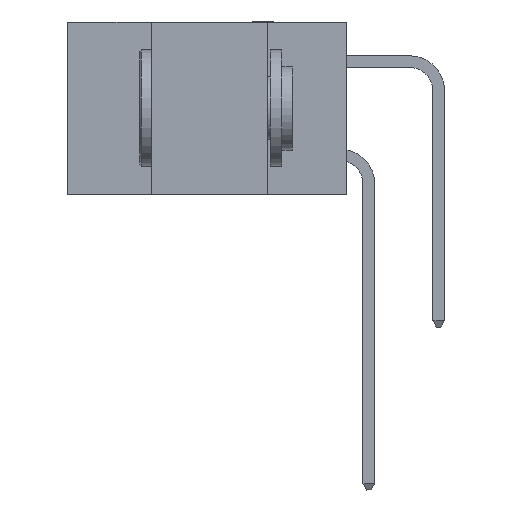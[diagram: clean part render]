
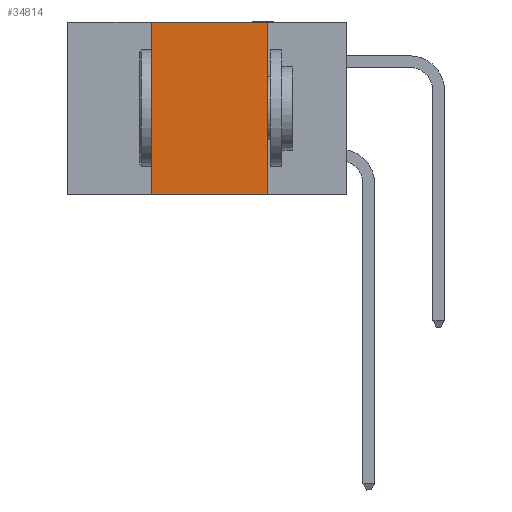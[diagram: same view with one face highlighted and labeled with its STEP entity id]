
A CAD part, left-side view. The second image highlights one B-rep face of the part: STEP entity #34814.
In plain terms, the highlighted planar face has unit normal (-1, 0, 0).
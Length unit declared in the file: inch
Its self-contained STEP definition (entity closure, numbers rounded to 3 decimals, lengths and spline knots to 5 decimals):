
#4759 = CARTESIAN_POINT ( 'NONE',  ( 0., 0.42, -0.37 ) ) ;
#5183 = VERTEX_POINT ( 'NONE', #14195 ) ;
#7444 = EDGE_CURVE ( 'NONE', #23126, #5183, #34120, .T. ) ;
#9278 = ORIENTED_EDGE ( 'NONE', *, *, #34131, .T. ) ;
#10661 = ORIENTED_EDGE ( 'NONE', *, *, #11235, .F. ) ;
#11235 = EDGE_CURVE ( 'NONE', #43028, #21261, #43667, .T. ) ;
#12449 = CARTESIAN_POINT ( 'NONE',  ( 0., 0.6, -0.37 ) ) ;
#12521 = CARTESIAN_POINT ( 'NONE',  ( 0., 0.6, 0. ) ) ;
#12543 = ORIENTED_EDGE ( 'NONE', *, *, #41556, .F. ) ;
#12591 = DIRECTION ( 'NONE',  ( 0., -1., 0. ) ) ;
#14195 = CARTESIAN_POINT ( 'NONE',  ( 0., 0.42, 0. ) ) ;
#14904 = LINE ( 'NONE', #12449, #32244 ) ;
#15912 = PLANE ( 'NONE',  #23015 ) ;
#16789 = VECTOR ( 'NONE', #43721, 39.37008 ) ;
#19611 = CARTESIAN_POINT ( 'NONE',  ( 0., 0.42, 0. ) ) ;
#20829 = DIRECTION ( 'NONE',  ( 0., 0., -1. ) ) ;
#21261 = VERTEX_POINT ( 'NONE', #26397 ) ;
#23015 = AXIS2_PLACEMENT_3D ( 'NONE', #12521, #43738, #23123 ) ;
#23018 = DIRECTION ( 'NONE',  ( 0., -1., 0. ) ) ;
#23123 = DIRECTION ( 'NONE',  ( 0., 0., -1. ) ) ;
#23126 = VERTEX_POINT ( 'NONE', #4759 ) ;
#25354 = VECTOR ( 'NONE', #20829, 39.37008 ) ;
#25921 = VECTOR ( 'NONE', #23018, 39.37008 ) ;
#26397 = CARTESIAN_POINT ( 'NONE',  ( 0., 0.17, -0.37 ) ) ;
#26781 = CARTESIAN_POINT ( 'NONE',  ( 0., 0.17, 0. ) ) ;
#32244 = VECTOR ( 'NONE', #12591, 39.37008 ) ;
#32946 = ORIENTED_EDGE ( 'NONE', *, *, #7444, .F. ) ;
#34120 = LINE ( 'NONE', #19611, #16789 ) ;
#34131 = EDGE_CURVE ( 'NONE', #23126, #21261, #14904, .T. ) ;
#34814 = ADVANCED_FACE ( 'NONE', ( #42991 ), #15912, .F. ) ;
#41435 = EDGE_LOOP ( 'NONE', ( #10661, #12543, #32946, #9278 ) ) ;
#41556 = EDGE_CURVE ( 'NONE', #5183, #43028, #43153, .T. ) ;
#42991 = FACE_OUTER_BOUND ( 'NONE', #41435, .T. ) ;
#43028 = VERTEX_POINT ( 'NONE', #26781 ) ;
#43153 = LINE ( 'NONE', #43619, #25921 ) ;
#43619 = CARTESIAN_POINT ( 'NONE',  ( 0., 0.6, 0. ) ) ;
#43667 = LINE ( 'NONE', #44914, #25354 ) ;
#43721 = DIRECTION ( 'NONE',  ( 0., 0., 1. ) ) ;
#43738 = DIRECTION ( 'NONE',  ( 1., 0., 0. ) ) ;
#44914 = CARTESIAN_POINT ( 'NONE',  ( 0., 0.17, 0. ) ) ;
